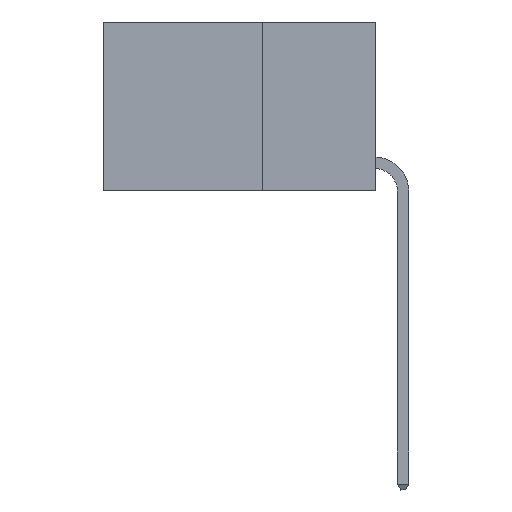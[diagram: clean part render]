
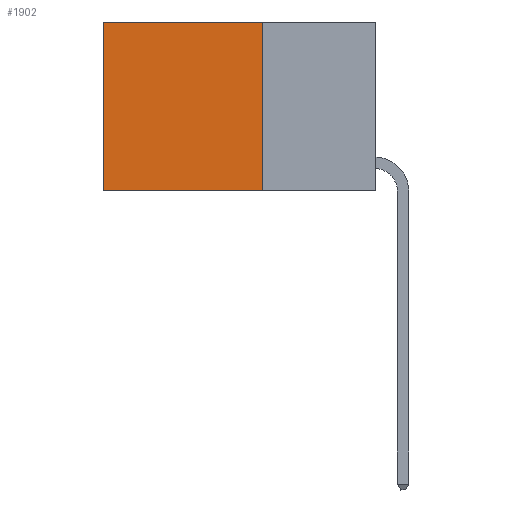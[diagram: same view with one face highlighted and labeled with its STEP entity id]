
A CAD part, left-side view. The second image highlights one B-rep face of the part: STEP entity #1902.
In plain terms, the highlighted planar face has unit normal (-1, 0, 0).
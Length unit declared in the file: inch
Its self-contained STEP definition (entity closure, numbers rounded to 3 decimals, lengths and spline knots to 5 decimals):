
#1447 = VECTOR ( 'NONE', #13065, 39.37008 ) ;
#1902 = ADVANCED_FACE ( 'NONE', ( #10496 ), #16289, .F. ) ;
#3072 = ORIENTED_EDGE ( 'NONE', *, *, #11532, .T. ) ;
#3173 = VERTEX_POINT ( 'NONE', #7534 ) ;
#3476 = EDGE_CURVE ( 'NONE', #11194, #17360, #6875, .T. ) ;
#4408 = EDGE_CURVE ( 'NONE', #3173, #16260, #5580, .T. ) ;
#4632 = VECTOR ( 'NONE', #13088, 39.37008 ) ;
#5556 = LINE ( 'NONE', #8480, #15740 ) ;
#5580 = LINE ( 'NONE', #8410, #1447 ) ;
#5788 = EDGE_CURVE ( 'NONE', #17360, #16260, #14713, .T. ) ;
#6291 = VECTOR ( 'NONE', #14393, 39.37008 ) ;
#6512 = CARTESIAN_POINT ( 'NONE',  ( 0.2625, 0.25, 0. ) ) ;
#6875 = LINE ( 'NONE', #8572, #6291 ) ;
#7534 = CARTESIAN_POINT ( 'NONE',  ( 0.2625, 0.6, 0. ) ) ;
#8410 = CARTESIAN_POINT ( 'NONE',  ( 0.2625, 0.6, 0. ) ) ;
#8480 = CARTESIAN_POINT ( 'NONE',  ( 0.2625, 0.25, 0. ) ) ;
#8572 = CARTESIAN_POINT ( 'NONE',  ( 0.2625, 0.25, 0. ) ) ;
#10271 = ORIENTED_EDGE ( 'NONE', *, *, #3476, .F. ) ;
#10496 = FACE_OUTER_BOUND ( 'NONE', #10845, .T. ) ;
#10845 = EDGE_LOOP ( 'NONE', ( #14119, #18315, #10271, #3072 ) ) ;
#11194 = VERTEX_POINT ( 'NONE', #12902 ) ;
#11341 = DIRECTION ( 'NONE',  ( 0., 1., 0. ) ) ;
#11532 = EDGE_CURVE ( 'NONE', #11194, #3173, #5556, .T. ) ;
#11928 = DIRECTION ( 'NONE',  ( 1., 0., 0. ) ) ;
#12312 = DIRECTION ( 'NONE',  ( 0., 0., -1. ) ) ;
#12902 = CARTESIAN_POINT ( 'NONE',  ( 0.2625, 0.25, 0. ) ) ;
#12988 = CARTESIAN_POINT ( 'NONE',  ( 0.2625, 0.6, -0.37 ) ) ;
#13065 = DIRECTION ( 'NONE',  ( 0., 0., -1. ) ) ;
#13088 = DIRECTION ( 'NONE',  ( 0., 1., 0. ) ) ;
#14119 = ORIENTED_EDGE ( 'NONE', *, *, #4408, .T. ) ;
#14393 = DIRECTION ( 'NONE',  ( 0., 0., -1. ) ) ;
#14713 = LINE ( 'NONE', #15846, #4632 ) ;
#15740 = VECTOR ( 'NONE', #11341, 39.37008 ) ;
#15846 = CARTESIAN_POINT ( 'NONE',  ( 0.2625, 0.25, -0.37 ) ) ;
#16260 = VERTEX_POINT ( 'NONE', #12988 ) ;
#16289 = PLANE ( 'NONE',  #18267 ) ;
#17191 = CARTESIAN_POINT ( 'NONE',  ( 0.2625, 0.25, -0.37 ) ) ;
#17360 = VERTEX_POINT ( 'NONE', #17191 ) ;
#18267 = AXIS2_PLACEMENT_3D ( 'NONE', #6512, #11928, #12312 ) ;
#18315 = ORIENTED_EDGE ( 'NONE', *, *, #5788, .F. ) ;
